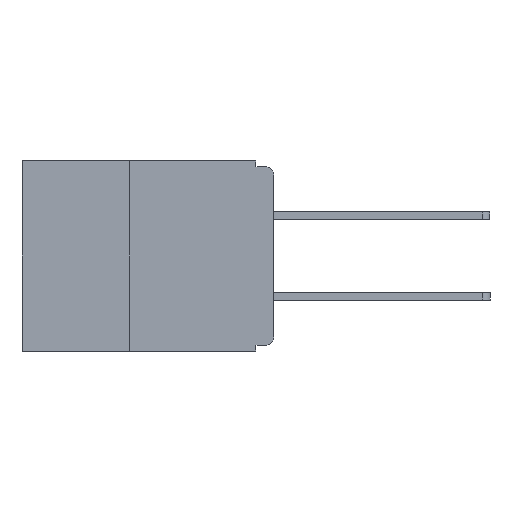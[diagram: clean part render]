
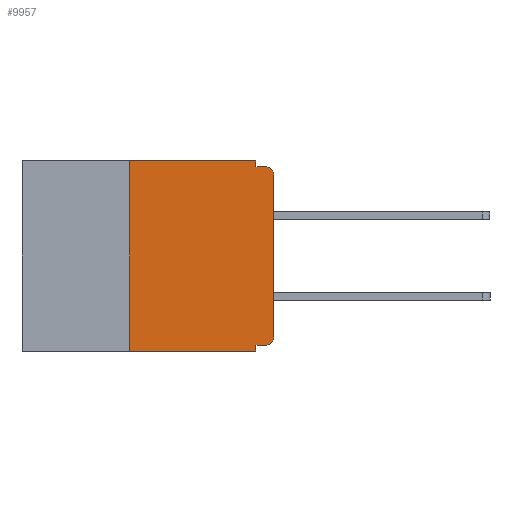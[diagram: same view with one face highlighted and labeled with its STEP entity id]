
A CAD part, left-side view. The second image highlights one B-rep face of the part: STEP entity #9957.
In plain terms, the highlighted planar face has unit normal (-1, 0, 0).
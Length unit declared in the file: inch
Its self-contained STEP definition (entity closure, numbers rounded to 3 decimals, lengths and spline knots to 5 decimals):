
#7 = FACE_OUTER_BOUND ( 'NONE', #22852, .T. ) ;
#303 = CARTESIAN_POINT ( 'NONE',  ( 0., 0.25, 0. ) ) ;
#342 = VECTOR ( 'NONE', #3948, 39.37008 ) ;
#720 = EDGE_CURVE ( 'NONE', #11851, #12817, #5035, .T. ) ;
#1140 = CIRCLE ( 'NONE', #3292, 0.015 ) ;
#1232 = ORIENTED_EDGE ( 'NONE', *, *, #5437, .F. ) ;
#2105 = CARTESIAN_POINT ( 'NONE',  ( 0., 0.25, -0.33 ) ) ;
#3093 = CARTESIAN_POINT ( 'NONE',  ( 0., 0.437, 0. ) ) ;
#3254 = EDGE_CURVE ( 'NONE', #10482, #13268, #3457, .T. ) ;
#3292 = AXIS2_PLACEMENT_3D ( 'NONE', #19909, #9273, #21663 ) ;
#3457 = LINE ( 'NONE', #17686, #8320 ) ;
#3948 = DIRECTION ( 'NONE',  ( 0., 0., 1. ) ) ;
#4199 = CARTESIAN_POINT ( 'NONE',  ( 0., 0.031, 0. ) ) ;
#5035 = CIRCLE ( 'NONE', #22379, 0.015 ) ;
#5084 = LINE ( 'NONE', #13733, #9390 ) ;
#5299 = CARTESIAN_POINT ( 'NONE',  ( 0., 0.031, 0. ) ) ;
#5437 = EDGE_CURVE ( 'NONE', #19968, #13268, #5084, .T. ) ;
#5546 = CARTESIAN_POINT ( 'NONE',  ( 0., 0.015, -0.01 ) ) ;
#5555 = VERTEX_POINT ( 'NONE', #12571 ) ;
#5901 = CARTESIAN_POINT ( 'NONE',  ( 0., 0., -0.01 ) ) ;
#6344 = ORIENTED_EDGE ( 'NONE', *, *, #7273, .F. ) ;
#6734 = DIRECTION ( 'NONE',  ( 0., -1., 0. ) ) ;
#7273 = EDGE_CURVE ( 'NONE', #17305, #12817, #17948, .T. ) ;
#7827 = CARTESIAN_POINT ( 'NONE',  ( 0., 0.031, -0.01 ) ) ;
#8320 = VECTOR ( 'NONE', #12251, 39.37008 ) ;
#8408 = ORIENTED_EDGE ( 'NONE', *, *, #3254, .T. ) ;
#8551 = CARTESIAN_POINT ( 'NONE',  ( 0., 0.031, -0.33 ) ) ;
#9187 = VECTOR ( 'NONE', #17774, 39.37008 ) ;
#9273 = DIRECTION ( 'NONE',  ( -1., 0., 0. ) ) ;
#9283 = ORIENTED_EDGE ( 'NONE', *, *, #12110, .F. ) ;
#9390 = VECTOR ( 'NONE', #13906, 39.37008 ) ;
#9957 = ADVANCED_FACE ( 'NONE', ( #7 ), #11592, .F. ) ;
#9958 = EDGE_CURVE ( 'NONE', #14203, #19968, #18634, .T. ) ;
#10092 = LINE ( 'NONE', #2105, #342 ) ;
#10217 = AXIS2_PLACEMENT_3D ( 'NONE', #11435, #10973, #11094 ) ;
#10469 = LINE ( 'NONE', #3093, #18756 ) ;
#10482 = VERTEX_POINT ( 'NONE', #16579 ) ;
#10623 = ORIENTED_EDGE ( 'NONE', *, *, #720, .T. ) ;
#10770 = CARTESIAN_POINT ( 'NONE',  ( 0., 0., -0.32 ) ) ;
#10820 = DIRECTION ( 'NONE',  ( 0., 1., 0. ) ) ;
#10973 = DIRECTION ( 'NONE',  ( 1., 0., 0. ) ) ;
#11094 = DIRECTION ( 'NONE',  ( 0., 0., -1. ) ) ;
#11435 = CARTESIAN_POINT ( 'NONE',  ( 0., 0.437, 0. ) ) ;
#11592 = PLANE ( 'NONE',  #10217 ) ;
#11851 = VERTEX_POINT ( 'NONE', #22040 ) ;
#12110 = EDGE_CURVE ( 'NONE', #22436, #12474, #10469, .T. ) ;
#12251 = DIRECTION ( 'NONE',  ( 0., -1., 0. ) ) ;
#12474 = VERTEX_POINT ( 'NONE', #4199 ) ;
#12571 = CARTESIAN_POINT ( 'NONE',  ( 0., 0., -0.305 ) ) ;
#12628 = DIRECTION ( 'NONE',  ( 0., 0., -1. ) ) ;
#12817 = VERTEX_POINT ( 'NONE', #5546 ) ;
#13268 = VERTEX_POINT ( 'NONE', #8551 ) ;
#13733 = CARTESIAN_POINT ( 'NONE',  ( 0., 0.031, -0.33 ) ) ;
#13906 = DIRECTION ( 'NONE',  ( 0., 0., -1. ) ) ;
#13983 = LINE ( 'NONE', #16015, #9187 ) ;
#14203 = VERTEX_POINT ( 'NONE', #16292 ) ;
#14509 = LINE ( 'NONE', #5299, #17529 ) ;
#14957 = DIRECTION ( 'NONE',  ( 0., 0., -1. ) ) ;
#15016 = CARTESIAN_POINT ( 'NONE',  ( 0., 0.015, -0.025 ) ) ;
#15409 = EDGE_CURVE ( 'NONE', #5555, #11851, #13983, .T. ) ;
#15633 = DIRECTION ( 'NONE',  ( -1., 0., 0. ) ) ;
#15648 = VECTOR ( 'NONE', #10820, 39.37008 ) ;
#16015 = CARTESIAN_POINT ( 'NONE',  ( 0., 0., 0. ) ) ;
#16292 = CARTESIAN_POINT ( 'NONE',  ( 0., 0.015, -0.32 ) ) ;
#16479 = ORIENTED_EDGE ( 'NONE', *, *, #17077, .F. ) ;
#16579 = CARTESIAN_POINT ( 'NONE',  ( 0., 0.25, -0.33 ) ) ;
#17077 = EDGE_CURVE ( 'NONE', #12474, #17305, #14509, .T. ) ;
#17305 = VERTEX_POINT ( 'NONE', #7827 ) ;
#17529 = VECTOR ( 'NONE', #12628, 39.37008 ) ;
#17686 = CARTESIAN_POINT ( 'NONE',  ( 0., 0.437, -0.33 ) ) ;
#17774 = DIRECTION ( 'NONE',  ( 0., 0., 1. ) ) ;
#17948 = LINE ( 'NONE', #5901, #22632 ) ;
#18306 = CARTESIAN_POINT ( 'NONE',  ( 0., 0.031, -0.32 ) ) ;
#18634 = LINE ( 'NONE', #10770, #15648 ) ;
#18722 = ORIENTED_EDGE ( 'NONE', *, *, #21230, .F. ) ;
#18756 = VECTOR ( 'NONE', #22804, 39.37008 ) ;
#19909 = CARTESIAN_POINT ( 'NONE',  ( 0., 0.015, -0.305 ) ) ;
#19968 = VERTEX_POINT ( 'NONE', #18306 ) ;
#21230 = EDGE_CURVE ( 'NONE', #10482, #22436, #10092, .T. ) ;
#21374 = ORIENTED_EDGE ( 'NONE', *, *, #15409, .T. ) ;
#21663 = DIRECTION ( 'NONE',  ( 0., 0., -1. ) ) ;
#21748 = ORIENTED_EDGE ( 'NONE', *, *, #9958, .F. ) ;
#22040 = CARTESIAN_POINT ( 'NONE',  ( 0., 0., -0.025 ) ) ;
#22300 = ORIENTED_EDGE ( 'NONE', *, *, #22337, .T. ) ;
#22337 = EDGE_CURVE ( 'NONE', #14203, #5555, #1140, .T. ) ;
#22379 = AXIS2_PLACEMENT_3D ( 'NONE', #15016, #15633, #14957 ) ;
#22436 = VERTEX_POINT ( 'NONE', #303 ) ;
#22632 = VECTOR ( 'NONE', #6734, 39.37008 ) ;
#22804 = DIRECTION ( 'NONE',  ( 0., -1., 0. ) ) ;
#22852 = EDGE_LOOP ( 'NONE', ( #21374, #10623, #6344, #16479, #9283, #18722, #8408, #1232, #21748, #22300 ) ) ;
